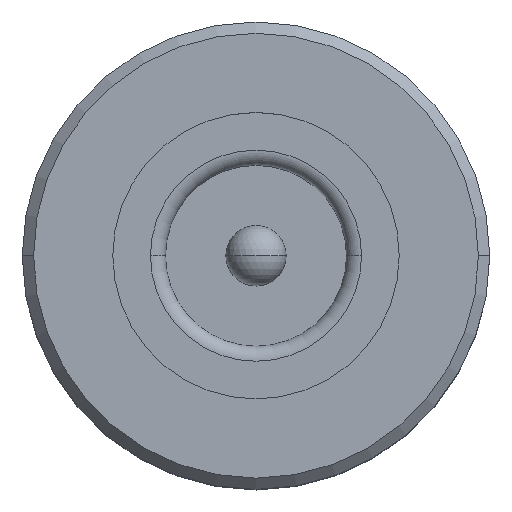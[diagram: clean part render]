
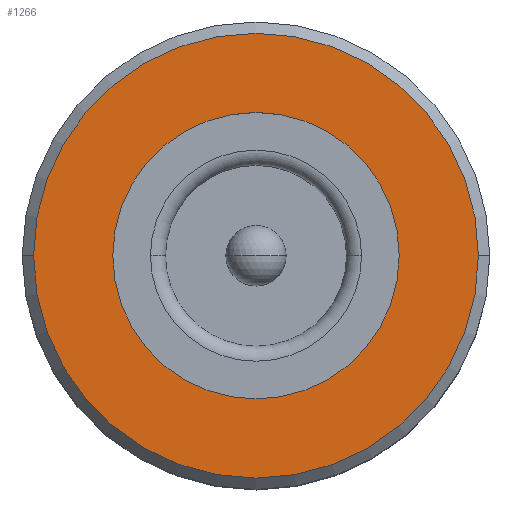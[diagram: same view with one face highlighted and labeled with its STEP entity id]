
A CAD part, top view. The second image highlights one B-rep face of the part: STEP entity #1266.
In plain terms, the highlighted planar face has unit normal (0, 0, 1).
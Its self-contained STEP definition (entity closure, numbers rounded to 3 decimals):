
#37 = CIRCLE ( 'NONE', #1096, 1.9 ) ;
#101 = EDGE_CURVE ( 'NONE', #447, #1613, #952, .T. ) ;
#138 = CARTESIAN_POINT ( 'NONE',  ( 60., -61.9, -6. ) ) ;
#149 = EDGE_CURVE ( 'NONE', #402, #1795, #37, .T. ) ;
#166 = EDGE_CURVE ( 'NONE', #1613, #447, #1774, .T. ) ;
#294 = CARTESIAN_POINT ( 'NONE',  ( 60., -60., -6. ) ) ;
#336 = AXIS2_PLACEMENT_3D ( 'NONE', #1161, #650, #1344 ) ;
#402 = VERTEX_POINT ( 'NONE', #1146 ) ;
#411 = DIRECTION ( 'NONE',  ( 0., 0., 1. ) ) ;
#413 = DIRECTION ( 'NONE',  ( 0., 0., 1. ) ) ;
#420 = DIRECTION ( 'NONE',  ( 1., 0., 0. ) ) ;
#447 = VERTEX_POINT ( 'NONE', #506 ) ;
#506 = CARTESIAN_POINT ( 'NONE',  ( 57.05, -60., -6. ) ) ;
#536 = CARTESIAN_POINT ( 'NONE',  ( 60., -60., -6. ) ) ;
#558 = FACE_BOUND ( 'NONE', #1260, .T. ) ;
#574 = CIRCLE ( 'NONE', #336, 1.9 ) ;
#613 = ORIENTED_EDGE ( 'NONE', *, *, #149, .F. ) ;
#650 = DIRECTION ( 'NONE',  ( 0., 0., -1. ) ) ;
#705 = DIRECTION ( 'NONE',  ( 0., 0., -1. ) ) ;
#820 = EDGE_CURVE ( 'NONE', #402, #1795, #574, .T. ) ;
#918 = AXIS2_PLACEMENT_3D ( 'NONE', #536, #705, #420 ) ;
#919 = ORIENTED_EDGE ( 'NONE', *, *, #101, .F. ) ;
#952 = CIRCLE ( 'NONE', #1230, 2.95 ) ;
#982 = CARTESIAN_POINT ( 'NONE',  ( 62.95, -60., -6. ) ) ;
#1035 = DIRECTION ( 'NONE',  ( 1., 0., 0. ) ) ;
#1096 = AXIS2_PLACEMENT_3D ( 'NONE', #1224, #411, #1612 ) ;
#1100 = DIRECTION ( 'NONE',  ( 0., 0., -1. ) ) ;
#1118 = ORIENTED_EDGE ( 'NONE', *, *, #166, .F. ) ;
#1146 = CARTESIAN_POINT ( 'NONE',  ( 60., -58.1, -6. ) ) ;
#1161 = CARTESIAN_POINT ( 'NONE',  ( 60., -60., -6. ) ) ;
#1196 = PLANE ( 'NONE',  #1271 ) ;
#1224 = CARTESIAN_POINT ( 'NONE',  ( 60., -60., -6. ) ) ;
#1230 = AXIS2_PLACEMENT_3D ( 'NONE', #294, #1100, #1987 ) ;
#1260 = EDGE_LOOP ( 'NONE', ( #613, #1316 ) ) ;
#1266 = ADVANCED_FACE ( 'NONE', ( #1961, #558 ), #1196, .T. ) ;
#1271 = AXIS2_PLACEMENT_3D ( 'NONE', #1803, #413, #1035 ) ;
#1316 = ORIENTED_EDGE ( 'NONE', *, *, #820, .T. ) ;
#1344 = DIRECTION ( 'NONE',  ( 0., 1., 0. ) ) ;
#1450 = EDGE_LOOP ( 'NONE', ( #1118, #919 ) ) ;
#1612 = DIRECTION ( 'NONE',  ( 0., 1., 0. ) ) ;
#1613 = VERTEX_POINT ( 'NONE', #982 ) ;
#1774 = CIRCLE ( 'NONE', #918, 2.95 ) ;
#1795 = VERTEX_POINT ( 'NONE', #138 ) ;
#1803 = CARTESIAN_POINT ( 'NONE',  ( 60., -60., -6. ) ) ;
#1961 = FACE_OUTER_BOUND ( 'NONE', #1450, .T. ) ;
#1987 = DIRECTION ( 'NONE',  ( -1., 0., 0. ) ) ;
